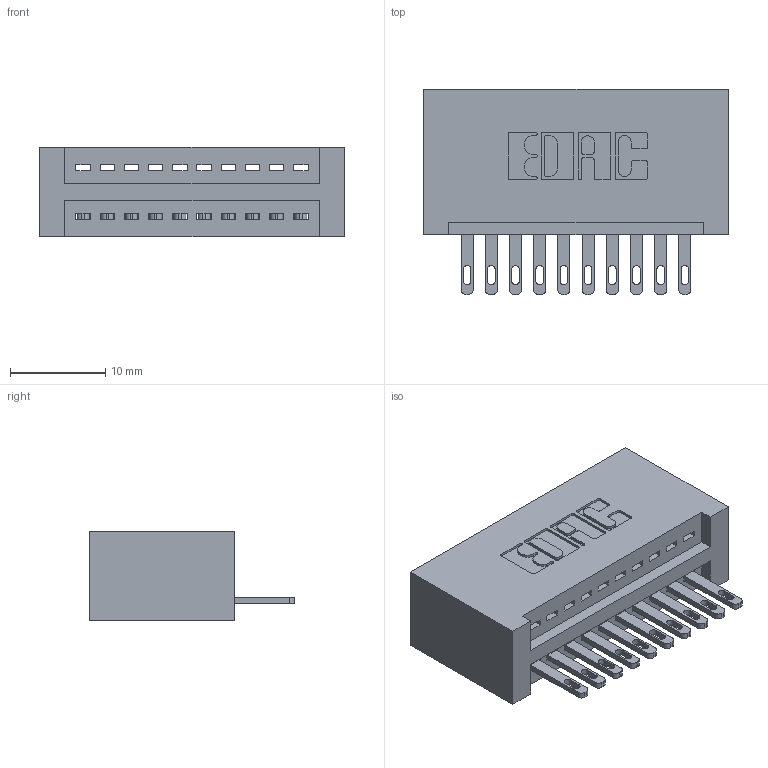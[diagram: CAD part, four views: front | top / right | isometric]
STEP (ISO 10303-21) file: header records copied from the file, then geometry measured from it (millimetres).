
FILE_DESCRIPTION (( 'STEP AP203' ), '1' );
FILE_NAME ('345-010-500-101.STEP', '2018-08-17T07:27:30', ( '' ), ( '' ), 'SwSTEP 2.0', 'SolidWorks 2016', '' );
FILE_SCHEMA (( 'CONFIG_CONTROL_DESIGN' ));
Length unit declared in the file: inch
Products named in the file (3): 345 Part_No Mounting Lugs; 345-292-001_345-293-100; 345-010-500-101
Assembly tree (11 placements, depth 2):
  345-010-500-101
    345 Part_No Mounting Lugs
    345-292-001_345-293-100  x10
Bounding box: 32 x 21.51 x 9.4 mm (x, y, z)
Volume: 3368.2 mm3; surface area: 4253.7 mm2
Topology: 11 solids, 11 shells, 658 faces, 1997 edges, 1330 vertices
Faces by surface type: plane 416, cylinder 242
Entity records: 11487 total; most frequent: CARTESIAN_POINT 1998, ORIENTED_EDGE 1942, DIRECTION 1787, EDGE_CURVE 971, LINE 803, VECTOR 803, VERTEX_POINT 646, AXIS2_PLACEMENT_3D 492
